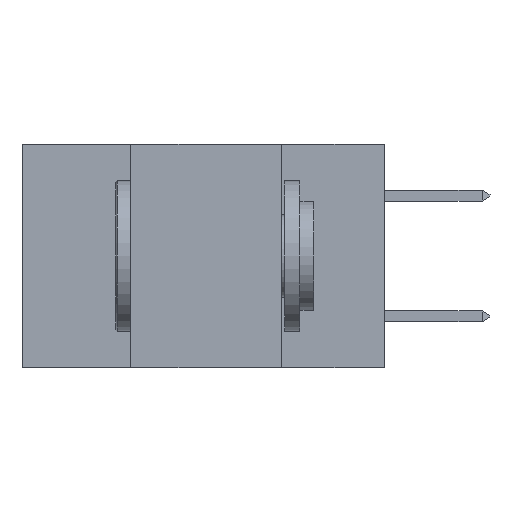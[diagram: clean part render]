
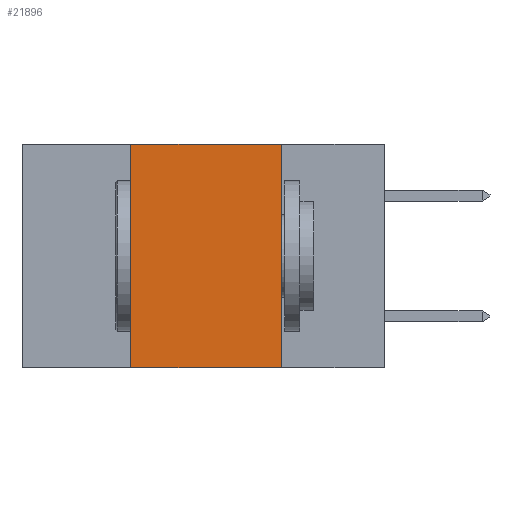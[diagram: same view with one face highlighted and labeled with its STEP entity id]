
A CAD part, left-side view. The second image highlights one B-rep face of the part: STEP entity #21896.
In plain terms, the highlighted planar face has unit normal (-1, 0, 0).
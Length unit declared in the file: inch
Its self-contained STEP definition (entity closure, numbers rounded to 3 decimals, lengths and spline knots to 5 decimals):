
#979 = VECTOR ( 'NONE', #1749, 39.37008 ) ;
#1749 = DIRECTION ( 'NONE',  ( 0., 0., 1. ) ) ;
#1827 = EDGE_CURVE ( 'NONE', #18675, #19778, #9585, .T. ) ;
#3030 = CARTESIAN_POINT ( 'NONE',  ( 0., 0.42, -0.37 ) ) ;
#3305 = CARTESIAN_POINT ( 'NONE',  ( 0., 0.17, 0. ) ) ;
#3601 = VECTOR ( 'NONE', #5107, 39.37008 ) ;
#4494 = VERTEX_POINT ( 'NONE', #3305 ) ;
#4558 = CARTESIAN_POINT ( 'NONE',  ( 0., 0.6, 0. ) ) ;
#5061 = VECTOR ( 'NONE', #11296, 39.37008 ) ;
#5107 = DIRECTION ( 'NONE',  ( 0., 0., -1. ) ) ;
#5240 = VECTOR ( 'NONE', #21542, 39.37008 ) ;
#5404 = EDGE_CURVE ( 'NONE', #19778, #4494, #21047, .T. ) ;
#7128 = DIRECTION ( 'NONE',  ( 0., 0., -1. ) ) ;
#8789 = ORIENTED_EDGE ( 'NONE', *, *, #1827, .F. ) ;
#9585 = LINE ( 'NONE', #17158, #979 ) ;
#10347 = DIRECTION ( 'NONE',  ( 1., 0., 0. ) ) ;
#11296 = DIRECTION ( 'NONE',  ( 0., -1., 0. ) ) ;
#12662 = CARTESIAN_POINT ( 'NONE',  ( 0., 0.17, -0.37 ) ) ;
#13970 = AXIS2_PLACEMENT_3D ( 'NONE', #22010, #10347, #7128 ) ;
#15524 = VERTEX_POINT ( 'NONE', #12662 ) ;
#15861 = CARTESIAN_POINT ( 'NONE',  ( 0., 0.6, -0.37 ) ) ;
#16412 = EDGE_CURVE ( 'NONE', #18675, #15524, #17687, .T. ) ;
#16432 = FACE_OUTER_BOUND ( 'NONE', #21111, .T. ) ;
#16597 = ORIENTED_EDGE ( 'NONE', *, *, #20474, .F. ) ;
#17158 = CARTESIAN_POINT ( 'NONE',  ( 0., 0.42, 0. ) ) ;
#17687 = LINE ( 'NONE', #15861, #5061 ) ;
#18110 = CARTESIAN_POINT ( 'NONE',  ( 0., 0.42, 0. ) ) ;
#18675 = VERTEX_POINT ( 'NONE', #3030 ) ;
#19145 = ORIENTED_EDGE ( 'NONE', *, *, #16412, .T. ) ;
#19778 = VERTEX_POINT ( 'NONE', #18110 ) ;
#20417 = ORIENTED_EDGE ( 'NONE', *, *, #5404, .F. ) ;
#20474 = EDGE_CURVE ( 'NONE', #4494, #15524, #21828, .T. ) ;
#21047 = LINE ( 'NONE', #4558, #5240 ) ;
#21111 = EDGE_LOOP ( 'NONE', ( #16597, #20417, #8789, #19145 ) ) ;
#21542 = DIRECTION ( 'NONE',  ( 0., -1., 0. ) ) ;
#21828 = LINE ( 'NONE', #21869, #3601 ) ;
#21869 = CARTESIAN_POINT ( 'NONE',  ( 0., 0.17, 0. ) ) ;
#21896 = ADVANCED_FACE ( 'NONE', ( #16432 ), #22162, .F. ) ;
#22010 = CARTESIAN_POINT ( 'NONE',  ( 0., 0.6, 0. ) ) ;
#22162 = PLANE ( 'NONE',  #13970 ) ;
